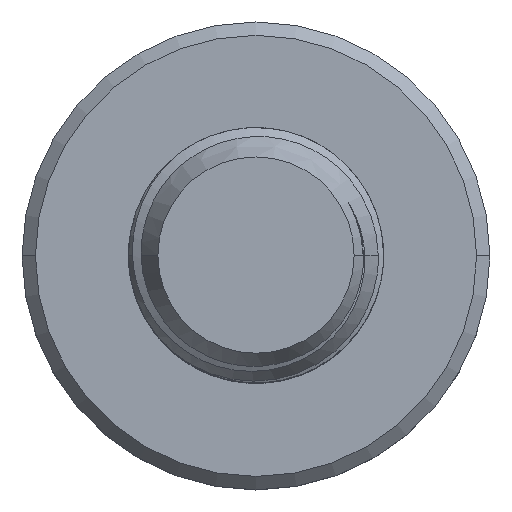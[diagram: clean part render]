
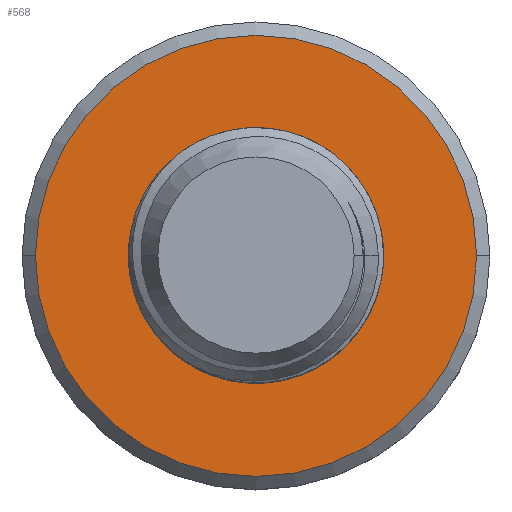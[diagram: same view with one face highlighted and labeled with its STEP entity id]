
A CAD part, top view. The second image highlights one B-rep face of the part: STEP entity #568.
In plain terms, the highlighted planar face has unit normal (0, 0, 1).
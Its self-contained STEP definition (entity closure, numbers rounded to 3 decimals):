
#128 = DIRECTION ( 'NONE',  ( 0., 0., 1. ) ) ;
#231 = CIRCLE ( 'NONE', #791, 3.293 ) ;
#273 = CARTESIAN_POINT ( 'NONE',  ( 0., 0., 0. ) ) ;
#348 = CIRCLE ( 'NONE', #1918, 1.905 ) ;
#377 = AXIS2_PLACEMENT_3D ( 'NONE', #1362, #128, #1582 ) ;
#439 = CARTESIAN_POINT ( 'NONE',  ( 1.905, 0., 0. ) ) ;
#465 = CARTESIAN_POINT ( 'NONE',  ( 3.293, 0., 0. ) ) ;
#487 = DIRECTION ( 'NONE',  ( 1., 0., 0. ) ) ;
#499 = ORIENTED_EDGE ( 'NONE', *, *, #2234, .T. ) ;
#568 = ADVANCED_FACE ( 'NONE', ( #1087, #2690 ), #2446, .F. ) ;
#722 = ORIENTED_EDGE ( 'NONE', *, *, #1410, .T. ) ;
#726 = DIRECTION ( 'NONE',  ( 0., 0., 1. ) ) ;
#791 = AXIS2_PLACEMENT_3D ( 'NONE', #1978, #726, #2207 ) ;
#819 = VERTEX_POINT ( 'NONE', #465 ) ;
#914 = ORIENTED_EDGE ( 'NONE', *, *, #2187, .F. ) ;
#919 = DIRECTION ( 'NONE',  ( 0., 0., 1. ) ) ;
#926 = CIRCLE ( 'NONE', #377, 3.293 ) ;
#933 = AXIS2_PLACEMENT_3D ( 'NONE', #2427, #2598, #2412 ) ;
#940 = VERTEX_POINT ( 'NONE', #1491 ) ;
#965 = ORIENTED_EDGE ( 'NONE', *, *, #2204, .F. ) ;
#1087 = FACE_OUTER_BOUND ( 'NONE', #2665, .T. ) ;
#1362 = CARTESIAN_POINT ( 'NONE',  ( 0., 0., 0. ) ) ;
#1389 = CIRCLE ( 'NONE', #2066, 1.905 ) ;
#1410 = EDGE_CURVE ( 'NONE', #819, #1998, #926, .T. ) ;
#1491 = CARTESIAN_POINT ( 'NONE',  ( -1.905, 0., 0. ) ) ;
#1582 = DIRECTION ( 'NONE',  ( -1., 0., 0. ) ) ;
#1741 = DIRECTION ( 'NONE',  ( 0., 0., 1. ) ) ;
#1918 = AXIS2_PLACEMENT_3D ( 'NONE', #2194, #919, #2419 ) ;
#1951 = CARTESIAN_POINT ( 'NONE',  ( -3.293, 0., 0. ) ) ;
#1978 = CARTESIAN_POINT ( 'NONE',  ( 0., 0., 0. ) ) ;
#1998 = VERTEX_POINT ( 'NONE', #1951 ) ;
#2066 = AXIS2_PLACEMENT_3D ( 'NONE', #273, #1741, #487 ) ;
#2138 = VERTEX_POINT ( 'NONE', #439 ) ;
#2187 = EDGE_CURVE ( 'NONE', #2138, #940, #348, .T. ) ;
#2194 = CARTESIAN_POINT ( 'NONE',  ( 0., 0., 0. ) ) ;
#2204 = EDGE_CURVE ( 'NONE', #940, #2138, #1389, .T. ) ;
#2207 = DIRECTION ( 'NONE',  ( -1., 0., 0. ) ) ;
#2234 = EDGE_CURVE ( 'NONE', #1998, #819, #231, .T. ) ;
#2331 = EDGE_LOOP ( 'NONE', ( #914, #965 ) ) ;
#2412 = DIRECTION ( 'NONE',  ( -1., 0., 0. ) ) ;
#2419 = DIRECTION ( 'NONE',  ( 1., 0., 0. ) ) ;
#2427 = CARTESIAN_POINT ( 'NONE',  ( 0., 1.905, 0. ) ) ;
#2446 = PLANE ( 'NONE',  #933 ) ;
#2598 = DIRECTION ( 'NONE',  ( 0., 0., -1. ) ) ;
#2665 = EDGE_LOOP ( 'NONE', ( #499, #722 ) ) ;
#2690 = FACE_BOUND ( 'NONE', #2331, .T. ) ;
